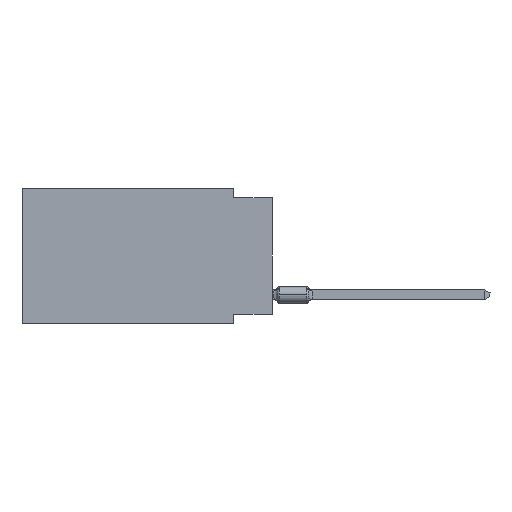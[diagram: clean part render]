
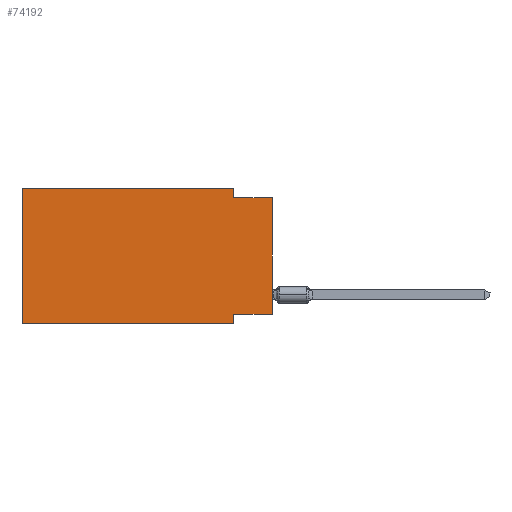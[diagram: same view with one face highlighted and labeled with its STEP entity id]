
A CAD part, left-side view. The second image highlights one B-rep face of the part: STEP entity #74192.
In plain terms, the highlighted planar face has unit normal (-1, 0, 0).
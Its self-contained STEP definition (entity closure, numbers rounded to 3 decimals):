
#557 = CARTESIAN_POINT ( 'NONE',  ( 0., 16.383, 0. ) ) ;
#1697 = EDGE_LOOP ( 'NONE', ( #3874, #31977, #73577, #72173, #6505, #83327, #38263, #15596 ) ) ;
#2258 = VERTEX_POINT ( 'NONE', #82634 ) ;
#3874 = ORIENTED_EDGE ( 'NONE', *, *, #19782, .T. ) ;
#4492 = VERTEX_POINT ( 'NONE', #33556 ) ;
#5267 = VERTEX_POINT ( 'NONE', #38148 ) ;
#5320 = AXIS2_PLACEMENT_3D ( 'NONE', #557, #73594, #14023 ) ;
#5712 = CARTESIAN_POINT ( 'NONE',  ( 0., 16.383, 0. ) ) ;
#5840 = LINE ( 'NONE', #80179, #39900 ) ;
#6173 = LINE ( 'NONE', #12685, #8570 ) ;
#6505 = ORIENTED_EDGE ( 'NONE', *, *, #67754, .F. ) ;
#6994 = LINE ( 'NONE', #38001, #65793 ) ;
#8570 = VECTOR ( 'NONE', #24872, 1000. ) ;
#10477 = DIRECTION ( 'NONE',  ( 0., 0., -1. ) ) ;
#12685 = CARTESIAN_POINT ( 'NONE',  ( 0., 0., -8.255 ) ) ;
#13223 = DIRECTION ( 'NONE',  ( 0., 0., 1. ) ) ;
#14023 = DIRECTION ( 'NONE',  ( 0., 0., -1. ) ) ;
#15189 = VERTEX_POINT ( 'NONE', #51921 ) ;
#15596 = ORIENTED_EDGE ( 'NONE', *, *, #16703, .F. ) ;
#16198 = LINE ( 'NONE', #56185, #68403 ) ;
#16703 = EDGE_CURVE ( 'NONE', #85464, #61768, #6173, .T. ) ;
#17854 = LINE ( 'NONE', #31315, #41178 ) ;
#18871 = DIRECTION ( 'NONE',  ( 0., -1., 0. ) ) ;
#19297 = CARTESIAN_POINT ( 'NONE',  ( 0., 0., -0.635 ) ) ;
#19782 = EDGE_CURVE ( 'NONE', #85464, #62894, #5840, .T. ) ;
#24872 = DIRECTION ( 'NONE',  ( 0., 1., 0. ) ) ;
#25611 = CARTESIAN_POINT ( 'NONE',  ( 0., 0., -8.255 ) ) ;
#26997 = LINE ( 'NONE', #5712, #46442 ) ;
#28440 = EDGE_CURVE ( 'NONE', #15189, #62894, #85402, .T. ) ;
#31182 = LINE ( 'NONE', #37700, #69422 ) ;
#31315 = CARTESIAN_POINT ( 'NONE',  ( 0., 2.54, 0. ) ) ;
#31977 = ORIENTED_EDGE ( 'NONE', *, *, #28440, .F. ) ;
#33556 = CARTESIAN_POINT ( 'NONE',  ( 0., 2.54, 0. ) ) ;
#33599 = FACE_OUTER_BOUND ( 'NONE', #1697, .T. ) ;
#36460 = EDGE_CURVE ( 'NONE', #2258, #4492, #26997, .T. ) ;
#37700 = CARTESIAN_POINT ( 'NONE',  ( 0., 16.383, -8.89 ) ) ;
#38001 = CARTESIAN_POINT ( 'NONE',  ( 0., 16.383, 0. ) ) ;
#38148 = CARTESIAN_POINT ( 'NONE',  ( 0., 2.54, -8.89 ) ) ;
#38263 = ORIENTED_EDGE ( 'NONE', *, *, #66032, .F. ) ;
#39900 = VECTOR ( 'NONE', #13223, 1000. ) ;
#41178 = VECTOR ( 'NONE', #10477, 1000. ) ;
#42706 = DIRECTION ( 'NONE',  ( 0., 0., -1. ) ) ;
#46442 = VECTOR ( 'NONE', #72229, 1000. ) ;
#50308 = VECTOR ( 'NONE', #18871, 1000. ) ;
#51050 = DIRECTION ( 'NONE',  ( 0., 0., 1. ) ) ;
#51921 = CARTESIAN_POINT ( 'NONE',  ( 0., 2.54, -0.635 ) ) ;
#54265 = CARTESIAN_POINT ( 'NONE',  ( 0., 16.383, -8.89 ) ) ;
#56185 = CARTESIAN_POINT ( 'NONE',  ( 0., 2.54, -8.89 ) ) ;
#58558 = DIRECTION ( 'NONE',  ( 0., -1., 0. ) ) ;
#59750 = CARTESIAN_POINT ( 'NONE',  ( 0., 2.54, -8.255 ) ) ;
#59857 = VERTEX_POINT ( 'NONE', #54265 ) ;
#61768 = VERTEX_POINT ( 'NONE', #59750 ) ;
#62086 = EDGE_CURVE ( 'NONE', #4492, #15189, #17854, .T. ) ;
#62894 = VERTEX_POINT ( 'NONE', #19297 ) ;
#65793 = VECTOR ( 'NONE', #51050, 1000. ) ;
#65812 = CARTESIAN_POINT ( 'NONE',  ( 0., 0., -0.635 ) ) ;
#66032 = EDGE_CURVE ( 'NONE', #61768, #5267, #16198, .T. ) ;
#67754 = EDGE_CURVE ( 'NONE', #59857, #2258, #6994, .T. ) ;
#68403 = VECTOR ( 'NONE', #42706, 1000. ) ;
#69422 = VECTOR ( 'NONE', #58558, 1000. ) ;
#72173 = ORIENTED_EDGE ( 'NONE', *, *, #36460, .F. ) ;
#72229 = DIRECTION ( 'NONE',  ( 0., -1., 0. ) ) ;
#72750 = PLANE ( 'NONE',  #5320 ) ;
#73577 = ORIENTED_EDGE ( 'NONE', *, *, #62086, .F. ) ;
#73594 = DIRECTION ( 'NONE',  ( 1., 0., 0. ) ) ;
#74192 = ADVANCED_FACE ( 'NONE', ( #33599 ), #72750, .F. ) ;
#77784 = EDGE_CURVE ( 'NONE', #59857, #5267, #31182, .T. ) ;
#80179 = CARTESIAN_POINT ( 'NONE',  ( 0., 0., 0. ) ) ;
#82634 = CARTESIAN_POINT ( 'NONE',  ( 0., 16.383, 0. ) ) ;
#83327 = ORIENTED_EDGE ( 'NONE', *, *, #77784, .T. ) ;
#85402 = LINE ( 'NONE', #65812, #50308 ) ;
#85464 = VERTEX_POINT ( 'NONE', #25611 ) ;
